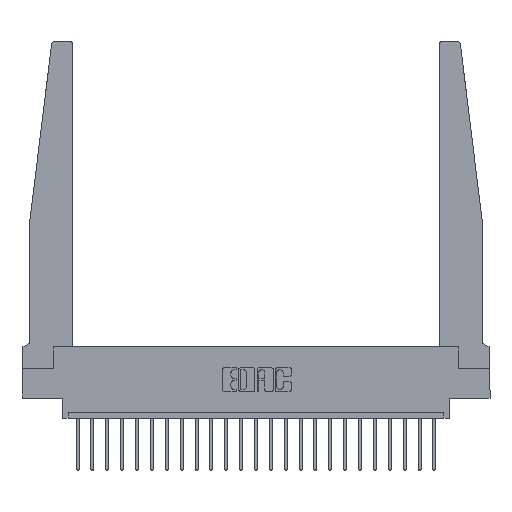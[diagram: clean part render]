
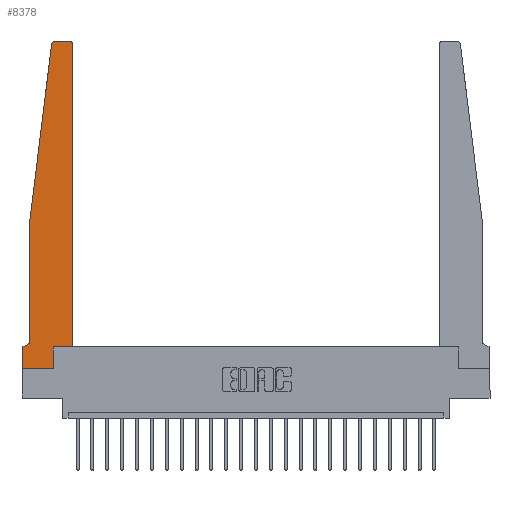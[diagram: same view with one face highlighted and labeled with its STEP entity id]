
A CAD part, top view. The second image highlights one B-rep face of the part: STEP entity #8378.
In plain terms, the highlighted planar face has unit normal (0, 0, 1).
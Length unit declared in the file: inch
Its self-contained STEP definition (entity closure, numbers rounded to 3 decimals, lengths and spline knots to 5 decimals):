
#19 = ORIENTED_EDGE ( 'NONE', *, *, #9576, .T. ) ;
#151 = CARTESIAN_POINT ( 'NONE',  ( 0.27653, 2.72, 0.37 ) ) ;
#363 = CARTESIAN_POINT ( 'NONE',  ( 0.395, 2.72, 0.37 ) ) ;
#455 = VERTEX_POINT ( 'NONE', #16746 ) ;
#503 = DIRECTION ( 'NONE',  ( 1., 0., 0. ) ) ;
#899 = DIRECTION ( 'NONE',  ( 0., 1., 0. ) ) ;
#929 = EDGE_CURVE ( 'NONE', #14596, #15482, #5805, .T. ) ;
#1286 = CARTESIAN_POINT ( 'NONE',  ( 0.2605, 0.18, 0.37 ) ) ;
#1337 = VECTOR ( 'NONE', #3807, 39.37008 ) ;
#1340 = DIRECTION ( 'NONE',  ( -1., 0., 0. ) ) ;
#1406 = CIRCLE ( 'NONE', #17474, 0.03 ) ;
#1643 = CIRCLE ( 'NONE', #6498, 0.05 ) ;
#1673 = VERTEX_POINT ( 'NONE', #17582 ) ;
#2232 = DIRECTION ( 'NONE',  ( 0., 0., 1. ) ) ;
#2461 = VERTEX_POINT ( 'NONE', #5264 ) ;
#2723 = VERTEX_POINT ( 'NONE', #4551 ) ;
#3110 = CARTESIAN_POINT ( 'NONE',  ( 0.015, 0.2375, 0.37 ) ) ;
#3807 = DIRECTION ( 'NONE',  ( -1., 0., 0. ) ) ;
#3818 = EDGE_CURVE ( 'NONE', #11446, #18056, #1643, .T. ) ;
#3858 = EDGE_LOOP ( 'NONE', ( #9572, #13999, #19958, #8182, #5145, #21955, #6896, #14385, #21307, #19, #19130, #10559 ) ) ;
#3881 = EDGE_CURVE ( 'NONE', #9956, #2461, #18814, .T. ) ;
#4164 = DIRECTION ( 'NONE',  ( 1., 0., 0. ) ) ;
#4284 = EDGE_CURVE ( 'NONE', #18029, #455, #22108, .T. ) ;
#4551 = CARTESIAN_POINT ( 'NONE',  ( 0.425, 0.18, 0.37 ) ) ;
#4586 = CARTESIAN_POINT ( 'NONE',  ( 0.425, 2.72, 0.37 ) ) ;
#5145 = ORIENTED_EDGE ( 'NONE', *, *, #3818, .T. ) ;
#5178 = LINE ( 'NONE', #17592, #16068 ) ;
#5264 = CARTESIAN_POINT ( 'NONE',  ( 0.24675, 2.72367, 0.37 ) ) ;
#5805 = LINE ( 'NONE', #16573, #11080 ) ;
#5819 = EDGE_CURVE ( 'NONE', #2461, #1673, #10754, .T. ) ;
#5942 = DIRECTION ( 'NONE',  ( 0., 1., 0. ) ) ;
#6498 = AXIS2_PLACEMENT_3D ( 'NONE', #3110, #19236, #1340 ) ;
#6896 = ORIENTED_EDGE ( 'NONE', *, *, #4284, .T. ) ;
#7099 = VECTOR ( 'NONE', #9230, 39.37008 ) ;
#8104 = LINE ( 'NONE', #20621, #1337 ) ;
#8182 = ORIENTED_EDGE ( 'NONE', *, *, #18088, .T. ) ;
#8378 = ADVANCED_FACE ( 'NONE', ( #12555 ), #15936, .T. ) ;
#8586 = CARTESIAN_POINT ( 'NONE',  ( 0., 0.1875, 0.37 ) ) ;
#8753 = CARTESIAN_POINT ( 'NONE',  ( 0.2605, 0., 0.37 ) ) ;
#9043 = DIRECTION ( 'NONE',  ( 0., -1., 0. ) ) ;
#9230 = DIRECTION ( 'NONE',  ( -0.122, -0.992, 0. ) ) ;
#9572 = ORIENTED_EDGE ( 'NONE', *, *, #9763, .T. ) ;
#9576 = EDGE_CURVE ( 'NONE', #15482, #2723, #18165, .T. ) ;
#9763 = EDGE_CURVE ( 'NONE', #11983, #9956, #16874, .T. ) ;
#9956 = VERTEX_POINT ( 'NONE', #20810 ) ;
#9987 = AXIS2_PLACEMENT_3D ( 'NONE', #23093, #21326, #19569 ) ;
#10559 = ORIENTED_EDGE ( 'NONE', *, *, #13147, .T. ) ;
#10683 = VECTOR ( 'NONE', #20853, 39.37008 ) ;
#10754 = LINE ( 'NONE', #19876, #7099 ) ;
#11080 = VECTOR ( 'NONE', #899, 39.37008 ) ;
#11446 = VERTEX_POINT ( 'NONE', #20993 ) ;
#11983 = VERTEX_POINT ( 'NONE', #17214 ) ;
#12378 = VECTOR ( 'NONE', #5942, 39.37008 ) ;
#12555 = FACE_OUTER_BOUND ( 'NONE', #3858, .T. ) ;
#13147 = EDGE_CURVE ( 'NONE', #14971, #11983, #1406, .T. ) ;
#13704 = CARTESIAN_POINT ( 'NONE',  ( 0.25, 2.75, 0.37 ) ) ;
#13882 = VECTOR ( 'NONE', #18462, 39.37008 ) ;
#13999 = ORIENTED_EDGE ( 'NONE', *, *, #3881, .T. ) ;
#14385 = ORIENTED_EDGE ( 'NONE', *, *, #17964, .T. ) ;
#14424 = VECTOR ( 'NONE', #503, 39.37008 ) ;
#14482 = LINE ( 'NONE', #18000, #12378 ) ;
#14517 = DIRECTION ( 'NONE',  ( 1., 0., 0. ) ) ;
#14542 = DIRECTION ( 'NONE',  ( 0., 0., 1. ) ) ;
#14596 = VERTEX_POINT ( 'NONE', #8753 ) ;
#14971 = VERTEX_POINT ( 'NONE', #4586 ) ;
#15482 = VERTEX_POINT ( 'NONE', #1286 ) ;
#15936 = PLANE ( 'NONE',  #9987 ) ;
#16061 = DIRECTION ( 'NONE',  ( 1., 0., 0. ) ) ;
#16068 = VECTOR ( 'NONE', #9043, 39.37008 ) ;
#16465 = CARTESIAN_POINT ( 'NONE',  ( 0., 0., 0.37 ) ) ;
#16573 = CARTESIAN_POINT ( 'NONE',  ( 0.2605, 0.18, 0.37 ) ) ;
#16746 = CARTESIAN_POINT ( 'NONE',  ( 0., 0., 0.37 ) ) ;
#16785 = CARTESIAN_POINT ( 'NONE',  ( 0., 0., 0.37 ) ) ;
#16874 = LINE ( 'NONE', #13704, #10683 ) ;
#17214 = CARTESIAN_POINT ( 'NONE',  ( 0.395, 2.75, 0.37 ) ) ;
#17474 = AXIS2_PLACEMENT_3D ( 'NONE', #363, #2232, #14517 ) ;
#17582 = CARTESIAN_POINT ( 'NONE',  ( 0.065, 1.25, 0.37 ) ) ;
#17592 = CARTESIAN_POINT ( 'NONE',  ( 0.065, 1.25, 0.37 ) ) ;
#17964 = EDGE_CURVE ( 'NONE', #455, #14596, #18540, .T. ) ;
#18000 = CARTESIAN_POINT ( 'NONE',  ( 0.425, 0.18, 0.37 ) ) ;
#18029 = VERTEX_POINT ( 'NONE', #8586 ) ;
#18056 = VERTEX_POINT ( 'NONE', #22513 ) ;
#18088 = EDGE_CURVE ( 'NONE', #1673, #11446, #5178, .T. ) ;
#18165 = LINE ( 'NONE', #19922, #14424 ) ;
#18462 = DIRECTION ( 'NONE',  ( 0., -1., 0. ) ) ;
#18540 = LINE ( 'NONE', #16785, #21703 ) ;
#18814 = CIRCLE ( 'NONE', #19190, 0.03 ) ;
#19090 = EDGE_CURVE ( 'NONE', #2723, #14971, #14482, .T. ) ;
#19130 = ORIENTED_EDGE ( 'NONE', *, *, #19090, .T. ) ;
#19190 = AXIS2_PLACEMENT_3D ( 'NONE', #151, #14542, #16061 ) ;
#19236 = DIRECTION ( 'NONE',  ( 0., 0., -1. ) ) ;
#19569 = DIRECTION ( 'NONE',  ( 1., 0., 0. ) ) ;
#19876 = CARTESIAN_POINT ( 'NONE',  ( 0.065, 1.25, 0.37 ) ) ;
#19922 = CARTESIAN_POINT ( 'NONE',  ( 0.425, 0.18, 0.37 ) ) ;
#19958 = ORIENTED_EDGE ( 'NONE', *, *, #5819, .T. ) ;
#20621 = CARTESIAN_POINT ( 'NONE',  ( 0.065, 0.1875, 0.37 ) ) ;
#20810 = CARTESIAN_POINT ( 'NONE',  ( 0.27653, 2.75, 0.37 ) ) ;
#20853 = DIRECTION ( 'NONE',  ( -1., 0., 0. ) ) ;
#20993 = CARTESIAN_POINT ( 'NONE',  ( 0.065, 0.2375, 0.37 ) ) ;
#21307 = ORIENTED_EDGE ( 'NONE', *, *, #929, .T. ) ;
#21326 = DIRECTION ( 'NONE',  ( 0., 0., 1. ) ) ;
#21703 = VECTOR ( 'NONE', #4164, 39.37008 ) ;
#21955 = ORIENTED_EDGE ( 'NONE', *, *, #23087, .T. ) ;
#22108 = LINE ( 'NONE', #16465, #13882 ) ;
#22513 = CARTESIAN_POINT ( 'NONE',  ( 0.015, 0.1875, 0.37 ) ) ;
#23087 = EDGE_CURVE ( 'NONE', #18056, #18029, #8104, .T. ) ;
#23093 = CARTESIAN_POINT ( 'NONE',  ( 0., 0.1875, 0.37 ) ) ;
